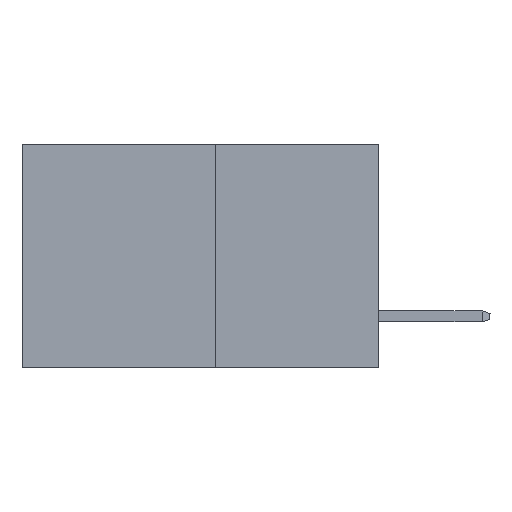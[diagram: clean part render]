
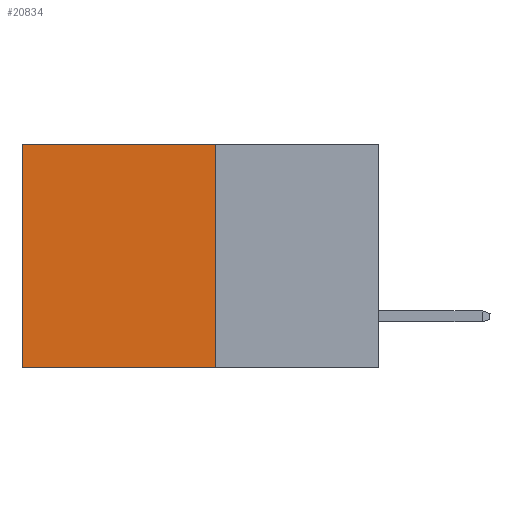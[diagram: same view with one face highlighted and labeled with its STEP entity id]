
A CAD part, left-side view. The second image highlights one B-rep face of the part: STEP entity #20834.
In plain terms, the highlighted planar face has unit normal (-1, 0, 0).
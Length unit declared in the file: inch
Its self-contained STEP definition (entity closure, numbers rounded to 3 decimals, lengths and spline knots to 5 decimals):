
#145 = LINE ( 'NONE', #895, #11317 ) ;
#458 = DIRECTION ( 'NONE',  ( 0., 0., -1. ) ) ;
#463 = AXIS2_PLACEMENT_3D ( 'NONE', #23636, #25694, #13212 ) ;
#895 = CARTESIAN_POINT ( 'NONE',  ( 0.277, 0.27, 0. ) ) ;
#960 = ORIENTED_EDGE ( 'NONE', *, *, #17370, .F. ) ;
#2528 = CARTESIAN_POINT ( 'NONE',  ( 0.277, 0.27, -0.37 ) ) ;
#3610 = DIRECTION ( 'NONE',  ( 0., 0., -1. ) ) ;
#4451 = EDGE_CURVE ( 'NONE', #26151, #11883, #145, .T. ) ;
#4534 = VECTOR ( 'NONE', #458, 39.37008 ) ;
#5128 = VERTEX_POINT ( 'NONE', #15631 ) ;
#5275 = FACE_OUTER_BOUND ( 'NONE', #19917, .T. ) ;
#8485 = CARTESIAN_POINT ( 'NONE',  ( 0.277, 0.27, -0.37 ) ) ;
#8822 = ORIENTED_EDGE ( 'NONE', *, *, #18992, .T. ) ;
#8981 = VERTEX_POINT ( 'NONE', #15755 ) ;
#10420 = ORIENTED_EDGE ( 'NONE', *, *, #14442, .F. ) ;
#10480 = LINE ( 'NONE', #20336, #26460 ) ;
#11317 = VECTOR ( 'NONE', #21918, 39.37008 ) ;
#11883 = VERTEX_POINT ( 'NONE', #17860 ) ;
#13212 = DIRECTION ( 'NONE',  ( 0., 0., -1. ) ) ;
#14442 = EDGE_CURVE ( 'NONE', #26151, #8981, #21337, .T. ) ;
#15631 = CARTESIAN_POINT ( 'NONE',  ( 0.277, 0.59, -0.37 ) ) ;
#15755 = CARTESIAN_POINT ( 'NONE',  ( 0.277, 0.27, -0.37 ) ) ;
#16127 = CARTESIAN_POINT ( 'NONE',  ( 0.277, 0.27, 0. ) ) ;
#16621 = ORIENTED_EDGE ( 'NONE', *, *, #4451, .T. ) ;
#17370 = EDGE_CURVE ( 'NONE', #8981, #5128, #25290, .T. ) ;
#17860 = CARTESIAN_POINT ( 'NONE',  ( 0.277, 0.59, 0. ) ) ;
#18992 = EDGE_CURVE ( 'NONE', #11883, #5128, #10480, .T. ) ;
#19723 = VECTOR ( 'NONE', #23195, 39.37008 ) ;
#19917 = EDGE_LOOP ( 'NONE', ( #8822, #960, #10420, #16621 ) ) ;
#20336 = CARTESIAN_POINT ( 'NONE',  ( 0.277, 0.59, -0.37 ) ) ;
#20834 = ADVANCED_FACE ( 'NONE', ( #5275 ), #21539, .F. ) ;
#21337 = LINE ( 'NONE', #2528, #4534 ) ;
#21539 = PLANE ( 'NONE',  #463 ) ;
#21918 = DIRECTION ( 'NONE',  ( 0., 1., 0. ) ) ;
#23195 = DIRECTION ( 'NONE',  ( 0., 1., 0. ) ) ;
#23636 = CARTESIAN_POINT ( 'NONE',  ( 0.277, 0.27, -0.37 ) ) ;
#25290 = LINE ( 'NONE', #8485, #19723 ) ;
#25694 = DIRECTION ( 'NONE',  ( 1., 0., 0. ) ) ;
#26151 = VERTEX_POINT ( 'NONE', #16127 ) ;
#26460 = VECTOR ( 'NONE', #3610, 39.37008 ) ;
